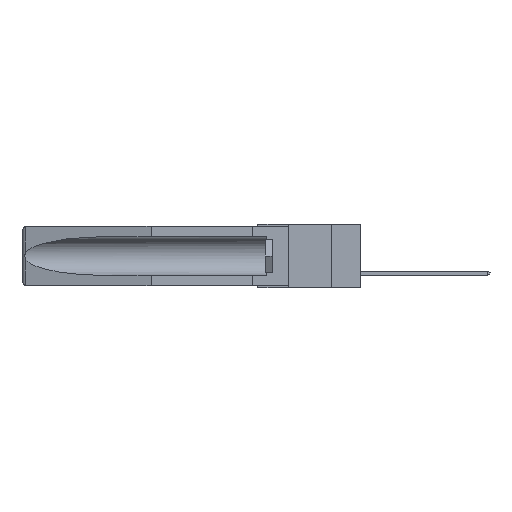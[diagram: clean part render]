
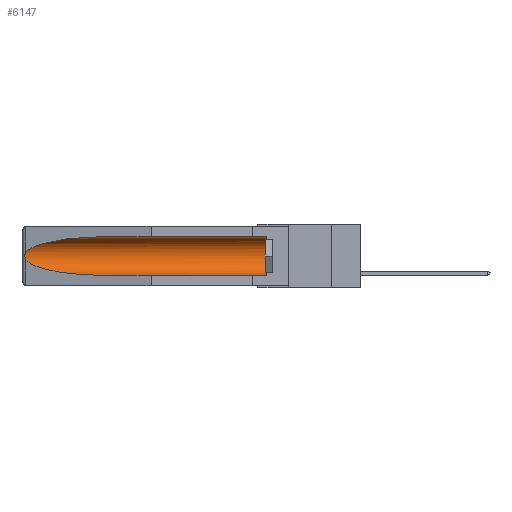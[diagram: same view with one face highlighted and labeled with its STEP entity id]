
A CAD part, left-side view. The second image highlights one B-rep face of the part: STEP entity #6147.
In plain terms, the highlighted cylindrical face has radius 2.857 mm (diameter 5.715 mm), a partial arc.
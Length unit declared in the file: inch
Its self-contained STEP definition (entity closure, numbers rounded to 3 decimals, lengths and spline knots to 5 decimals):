
#124 = CARTESIAN_POINT ( 'NONE',  ( 0.26537, 1.52718, -0.14972 ) ) ;
#360 = CARTESIAN_POINT ( 'NONE',  ( 0.26537, 1.52718, -0.19328 ) ) ;
#551 = ORIENTED_EDGE ( 'NONE', *, *, #13641, .T. ) ;
#694 = EDGE_CURVE ( 'NONE', #16057, #13131, #16636, .T. ) ;
#870 = CARTESIAN_POINT ( 'NONE',  ( 0.2673, 1.53269, -0.17917 ) ) ;
#911 = CARTESIAN_POINT ( 'NONE',  ( 0.155, 1.07973, -0.059 ) ) ;
#1137 = B_SPLINE_CURVE_WITH_KNOTS ( 'NONE', 3,
 ( #12067, #3669, #7909, #10541, #13496, #14717, #870, #5081, #2311, #12128 ),
 .UNSPECIFIED., .F., .F.,
 ( 4, 2, 2, 2, 4 ),
 ( 0., 0.00029, 0.00058, 0.00087, 0.00117 ),
 .UNSPECIFIED. ) ;
#1229 = FACE_OUTER_BOUND ( 'NONE', #3294, .T. ) ;
#1649 = LINE ( 'NONE', #11526, #14409 ) ;
#1737 = CARTESIAN_POINT ( 'NONE',  ( 0.21114, 1.30732, -0.059 ) ) ;
#1846 = CARTESIAN_POINT ( 'NONE',  ( 0.21114, 1.30732, -0.284 ) ) ;
#2114 = VERTEX_POINT ( 'NONE', #16521 ) ;
#2311 = CARTESIAN_POINT ( 'NONE',  ( 0.26597, 1.5296, -0.19026 ) ) ;
#2727 = CARTESIAN_POINT ( 'NONE',  ( 0.26537, 1.52718, -0.14972 ) ) ;
#3294 = EDGE_LOOP ( 'NONE', ( #17801, #551, #3491, #9577, #8413, #7043 ) ) ;
#3482 = VERTEX_POINT ( 'NONE', #2727 ) ;
#3491 = ORIENTED_EDGE ( 'NONE', *, *, #3499, .T. ) ;
#3499 = EDGE_CURVE ( 'NONE', #7694, #2114, #11302, .T. ) ;
#3669 = CARTESIAN_POINT ( 'NONE',  ( 0.26597, 1.52961, -0.15275 ) ) ;
#4647 = CARTESIAN_POINT ( 'NONE',  ( 0.25451, 1.48313, -0.09465 ) ) ;
#4990 =( BOUNDED_CURVE ( )  B_SPLINE_CURVE ( 3, ( #8727, #1737, #4647, #124 ),
 .UNSPECIFIED., .F., .F. ) 
 B_SPLINE_CURVE_WITH_KNOTS ( ( 4, 4 ),
 ( 4.71239, 6.08839 ),
 .UNSPECIFIED. ) 
 CURVE ( )  GEOMETRIC_REPRESENTATION_ITEM ( )  RATIONAL_B_SPLINE_CURVE ( ( 1., 0.848, 0.848, 1. ) ) 
 REPRESENTATION_ITEM ( '' )  );
#5081 = CARTESIAN_POINT ( 'NONE',  ( 0.26655, 1.53094, -0.18657 ) ) ;
#5170 = VERTEX_POINT ( 'NONE', #9821 ) ;
#5630 = CARTESIAN_POINT ( 'NONE',  ( 0.26537, 1.52718, -0.19328 ) ) ;
#6147 = ADVANCED_FACE ( 'NONE', ( #1229 ), #17765, .F. ) ;
#6645 = EDGE_CURVE ( 'NONE', #5170, #16057, #13769, .T. ) ;
#7043 = ORIENTED_EDGE ( 'NONE', *, *, #694, .T. ) ;
#7694 = VERTEX_POINT ( 'NONE', #360 ) ;
#7880 = CARTESIAN_POINT ( 'NONE',  ( 0.155, 1.07973, -0.284 ) ) ;
#7909 = CARTESIAN_POINT ( 'NONE',  ( 0.26654, 1.53092, -0.15636 ) ) ;
#8032 = AXIS2_PLACEMENT_3D ( 'NONE', #17987, #9513, #10959 ) ;
#8413 = ORIENTED_EDGE ( 'NONE', *, *, #6645, .T. ) ;
#8598 = CARTESIAN_POINT ( 'NONE',  ( 0.25451, 1.48313, -0.24835 ) ) ;
#8727 = CARTESIAN_POINT ( 'NONE',  ( 0.155, 1.07973, -0.059 ) ) ;
#9120 = VECTOR ( 'NONE', #11377, 39.37008 ) ;
#9129 = CARTESIAN_POINT ( 'NONE',  ( 0.155, 0.126, -0.059 ) ) ;
#9513 = DIRECTION ( 'NONE',  ( 0., 1., 0. ) ) ;
#9577 = ORIENTED_EDGE ( 'NONE', *, *, #13920, .F. ) ;
#9821 = CARTESIAN_POINT ( 'NONE',  ( 0.155, 0.126, -0.284 ) ) ;
#9835 = EDGE_CURVE ( 'NONE', #13131, #3482, #4990, .T. ) ;
#10541 = CARTESIAN_POINT ( 'NONE',  ( 0.2673, 1.5327, -0.16383 ) ) ;
#10959 = DIRECTION ( 'NONE',  ( 0., 0., 1. ) ) ;
#11302 =( BOUNDED_CURVE ( )  B_SPLINE_CURVE ( 3, ( #5630, #8598, #1846, #7880 ),
 .UNSPECIFIED., .F., .F. ) 
 B_SPLINE_CURVE_WITH_KNOTS ( ( 4, 4 ),
 ( 0.1948, 1.5708 ),
 .UNSPECIFIED. ) 
 CURVE ( )  GEOMETRIC_REPRESENTATION_ITEM ( )  RATIONAL_B_SPLINE_CURVE ( ( 1., 0.848, 0.848, 1. ) ) 
 REPRESENTATION_ITEM ( '' )  );
#11377 = DIRECTION ( 'NONE',  ( 0., 1., 0. ) ) ;
#11526 = CARTESIAN_POINT ( 'NONE',  ( 0.155, -0.30754, -0.284 ) ) ;
#12067 = CARTESIAN_POINT ( 'NONE',  ( 0.26537, 1.52718, -0.14972 ) ) ;
#12128 = CARTESIAN_POINT ( 'NONE',  ( 0.26537, 1.52718, -0.19328 ) ) ;
#12868 = AXIS2_PLACEMENT_3D ( 'NONE', #13690, #14857, #14978 ) ;
#12934 = DIRECTION ( 'NONE',  ( 0., 1., 0. ) ) ;
#13131 = VERTEX_POINT ( 'NONE', #911 ) ;
#13496 = CARTESIAN_POINT ( 'NONE',  ( 0.2675, 1.53308, -0.16763 ) ) ;
#13641 = EDGE_CURVE ( 'NONE', #3482, #7694, #1137, .T. ) ;
#13690 = CARTESIAN_POINT ( 'NONE',  ( 0.155, 0.126, -0.1715 ) ) ;
#13769 = CIRCLE ( 'NONE', #12868, 0.1125 ) ;
#13920 = EDGE_CURVE ( 'NONE', #5170, #2114, #1649, .T. ) ;
#14140 = CARTESIAN_POINT ( 'NONE',  ( 0.155, -0.30754, -0.059 ) ) ;
#14409 = VECTOR ( 'NONE', #12934, 39.37008 ) ;
#14717 = CARTESIAN_POINT ( 'NONE',  ( 0.2675, 1.53308, -0.17534 ) ) ;
#14857 = DIRECTION ( 'NONE',  ( 0., -1., 0. ) ) ;
#14978 = DIRECTION ( 'NONE',  ( 0., 0., 1. ) ) ;
#16057 = VERTEX_POINT ( 'NONE', #9129 ) ;
#16521 = CARTESIAN_POINT ( 'NONE',  ( 0.155, 1.07973, -0.284 ) ) ;
#16636 = LINE ( 'NONE', #14140, #9120 ) ;
#17765 = CYLINDRICAL_SURFACE ( 'NONE', #8032, 0.1125 ) ;
#17801 = ORIENTED_EDGE ( 'NONE', *, *, #9835, .T. ) ;
#17987 = CARTESIAN_POINT ( 'NONE',  ( 0.155, -0.30754, -0.1715 ) ) ;
